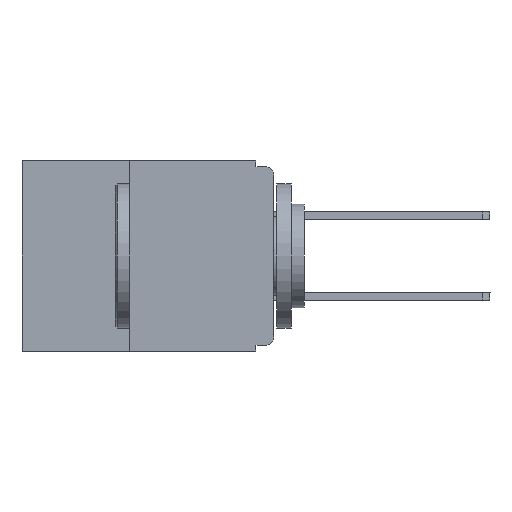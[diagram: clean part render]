
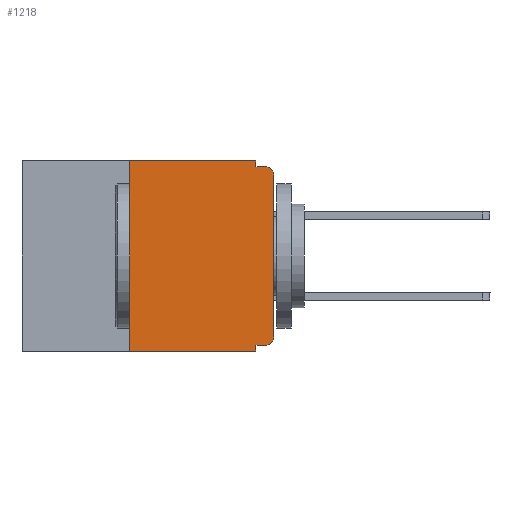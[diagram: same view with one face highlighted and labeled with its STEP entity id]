
A CAD part, left-side view. The second image highlights one B-rep face of the part: STEP entity #1218.
In plain terms, the highlighted planar face has unit normal (-1, 0, 0).
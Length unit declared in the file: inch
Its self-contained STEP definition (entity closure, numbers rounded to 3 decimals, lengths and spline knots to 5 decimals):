
#182 = VECTOR ( 'NONE', #9154, 39.37008 ) ;
#296 = VECTOR ( 'NONE', #4598, 39.37008 ) ;
#374 = ORIENTED_EDGE ( 'NONE', *, *, #5977, .F. ) ;
#437 = DIRECTION ( 'NONE',  ( 0., 1., 0. ) ) ;
#689 = EDGE_CURVE ( 'NONE', #6741, #10453, #9821, .T. ) ;
#763 = CARTESIAN_POINT ( 'NONE',  ( 0., 0.437, -0.33 ) ) ;
#913 = CARTESIAN_POINT ( 'NONE',  ( 0., 0.031, 0. ) ) ;
#1092 = VECTOR ( 'NONE', #11153, 39.37008 ) ;
#1193 = AXIS2_PLACEMENT_3D ( 'NONE', #8641, #5901, #6837 ) ;
#1218 = ADVANCED_FACE ( 'NONE', ( #6269 ), #8893, .F. ) ;
#1333 = CARTESIAN_POINT ( 'NONE',  ( 0., 0.437, 0. ) ) ;
#1739 = CARTESIAN_POINT ( 'NONE',  ( 0., 0.031, -0.01 ) ) ;
#1876 = EDGE_CURVE ( 'NONE', #6181, #2614, #7858, .T. ) ;
#2132 = LINE ( 'NONE', #9176, #4585 ) ;
#2270 = DIRECTION ( 'NONE',  ( 1., 0., 0. ) ) ;
#2614 = VERTEX_POINT ( 'NONE', #1739 ) ;
#2740 = DIRECTION ( 'NONE',  ( 0., 0., -1. ) ) ;
#2816 = ORIENTED_EDGE ( 'NONE', *, *, #1876, .F. ) ;
#3004 = CARTESIAN_POINT ( 'NONE',  ( 0., 0.25, -0.33 ) ) ;
#3037 = VECTOR ( 'NONE', #11994, 39.37008 ) ;
#3089 = DIRECTION ( 'NONE',  ( 0., 0., 1. ) ) ;
#3185 = LINE ( 'NONE', #4564, #3037 ) ;
#3276 = ORIENTED_EDGE ( 'NONE', *, *, #8946, .F. ) ;
#3506 = VECTOR ( 'NONE', #3633, 39.37008 ) ;
#3633 = DIRECTION ( 'NONE',  ( 0., 0., -1. ) ) ;
#3800 = ORIENTED_EDGE ( 'NONE', *, *, #4456, .T. ) ;
#3837 = EDGE_LOOP ( 'NONE', ( #8494, #11211, #374, #2816, #3276, #3861, #3800, #11428, #8255, #5039 ) ) ;
#3846 = VERTEX_POINT ( 'NONE', #8165 ) ;
#3861 = ORIENTED_EDGE ( 'NONE', *, *, #5537, .F. ) ;
#3995 = LINE ( 'NONE', #3004, #7785 ) ;
#4456 = EDGE_CURVE ( 'NONE', #3846, #4975, #5087, .T. ) ;
#4564 = CARTESIAN_POINT ( 'NONE',  ( 0., 0.437, 0. ) ) ;
#4585 = VECTOR ( 'NONE', #11900, 39.37008 ) ;
#4598 = DIRECTION ( 'NONE',  ( 0., 0., -1. ) ) ;
#4801 = VECTOR ( 'NONE', #437, 39.37008 ) ;
#4975 = VERTEX_POINT ( 'NONE', #10668 ) ;
#5039 = ORIENTED_EDGE ( 'NONE', *, *, #9268, .T. ) ;
#5087 = LINE ( 'NONE', #763, #182 ) ;
#5154 = CARTESIAN_POINT ( 'NONE',  ( 0., 0., -0.32 ) ) ;
#5537 = EDGE_CURVE ( 'NONE', #3846, #9432, #3995, .T. ) ;
#5555 = CARTESIAN_POINT ( 'NONE',  ( 0., 0.031, -0.33 ) ) ;
#5596 = CARTESIAN_POINT ( 'NONE',  ( 0., 0.015, -0.305 ) ) ;
#5689 = CARTESIAN_POINT ( 'NONE',  ( 0., 0.031, 0. ) ) ;
#5901 = DIRECTION ( 'NONE',  ( -1., 0., 0. ) ) ;
#5977 = EDGE_CURVE ( 'NONE', #2614, #9747, #2132, .T. ) ;
#6098 = LINE ( 'NONE', #5555, #296 ) ;
#6170 = VERTEX_POINT ( 'NONE', #8474 ) ;
#6181 = VERTEX_POINT ( 'NONE', #5689 ) ;
#6269 = FACE_OUTER_BOUND ( 'NONE', #3837, .T. ) ;
#6741 = VERTEX_POINT ( 'NONE', #7797 ) ;
#6837 = DIRECTION ( 'NONE',  ( 0., 0., -1. ) ) ;
#7230 = EDGE_CURVE ( 'NONE', #10453, #9747, #10389, .T. ) ;
#7388 = CARTESIAN_POINT ( 'NONE',  ( 0., 0., -0.025 ) ) ;
#7546 = CARTESIAN_POINT ( 'NONE',  ( 0., 0., 0. ) ) ;
#7785 = VECTOR ( 'NONE', #3089, 39.37008 ) ;
#7797 = CARTESIAN_POINT ( 'NONE',  ( 0., 0., -0.305 ) ) ;
#7858 = LINE ( 'NONE', #913, #3506 ) ;
#8165 = CARTESIAN_POINT ( 'NONE',  ( 0., 0.25, -0.33 ) ) ;
#8255 = ORIENTED_EDGE ( 'NONE', *, *, #8699, .F. ) ;
#8474 = CARTESIAN_POINT ( 'NONE',  ( 0., 0.015, -0.32 ) ) ;
#8494 = ORIENTED_EDGE ( 'NONE', *, *, #689, .T. ) ;
#8641 = CARTESIAN_POINT ( 'NONE',  ( 0., 0.015, -0.025 ) ) ;
#8675 = AXIS2_PLACEMENT_3D ( 'NONE', #5596, #11082, #2740 ) ;
#8699 = EDGE_CURVE ( 'NONE', #6170, #10778, #11220, .T. ) ;
#8893 = PLANE ( 'NONE',  #10992 ) ;
#8946 = EDGE_CURVE ( 'NONE', #9432, #6181, #3185, .T. ) ;
#9154 = DIRECTION ( 'NONE',  ( 0., -1., 0. ) ) ;
#9176 = CARTESIAN_POINT ( 'NONE',  ( 0., 0., -0.01 ) ) ;
#9268 = EDGE_CURVE ( 'NONE', #6170, #6741, #10911, .T. ) ;
#9328 = EDGE_CURVE ( 'NONE', #10778, #4975, #6098, .T. ) ;
#9340 = CARTESIAN_POINT ( 'NONE',  ( 0., 0.031, -0.32 ) ) ;
#9432 = VERTEX_POINT ( 'NONE', #11339 ) ;
#9747 = VERTEX_POINT ( 'NONE', #11043 ) ;
#9821 = LINE ( 'NONE', #7546, #1092 ) ;
#10389 = CIRCLE ( 'NONE', #1193, 0.015 ) ;
#10453 = VERTEX_POINT ( 'NONE', #7388 ) ;
#10668 = CARTESIAN_POINT ( 'NONE',  ( 0., 0.031, -0.33 ) ) ;
#10778 = VERTEX_POINT ( 'NONE', #9340 ) ;
#10911 = CIRCLE ( 'NONE', #8675, 0.015 ) ;
#10992 = AXIS2_PLACEMENT_3D ( 'NONE', #1333, #2270, #11663 ) ;
#11043 = CARTESIAN_POINT ( 'NONE',  ( 0., 0.015, -0.01 ) ) ;
#11082 = DIRECTION ( 'NONE',  ( -1., 0., 0. ) ) ;
#11153 = DIRECTION ( 'NONE',  ( 0., 0., 1. ) ) ;
#11211 = ORIENTED_EDGE ( 'NONE', *, *, #7230, .T. ) ;
#11220 = LINE ( 'NONE', #5154, #4801 ) ;
#11339 = CARTESIAN_POINT ( 'NONE',  ( 0., 0.25, 0. ) ) ;
#11428 = ORIENTED_EDGE ( 'NONE', *, *, #9328, .F. ) ;
#11663 = DIRECTION ( 'NONE',  ( 0., 0., -1. ) ) ;
#11900 = DIRECTION ( 'NONE',  ( 0., -1., 0. ) ) ;
#11994 = DIRECTION ( 'NONE',  ( 0., -1., 0. ) ) ;
